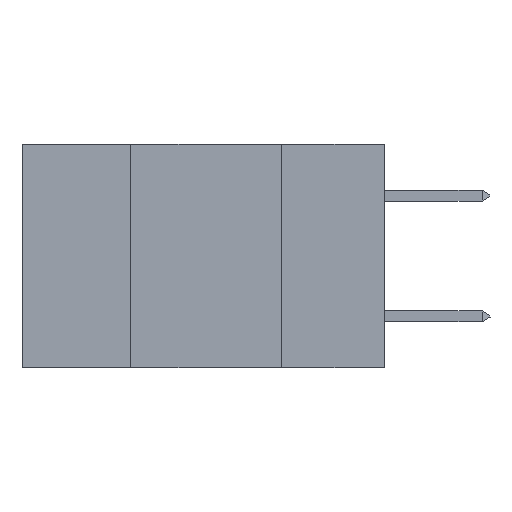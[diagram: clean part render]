
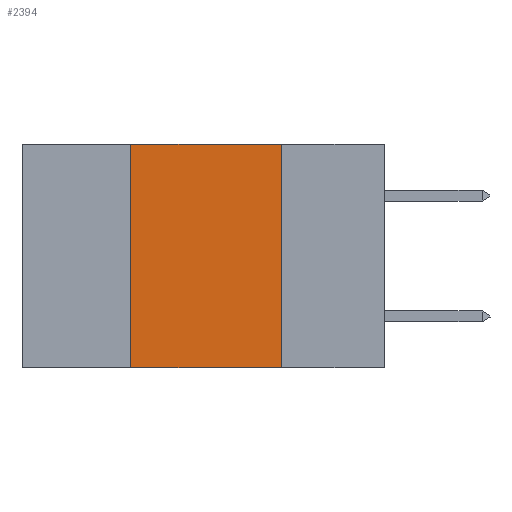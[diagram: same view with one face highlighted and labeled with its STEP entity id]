
A CAD part, left-side view. The second image highlights one B-rep face of the part: STEP entity #2394.
In plain terms, the highlighted planar face has unit normal (-1, 0, 0).
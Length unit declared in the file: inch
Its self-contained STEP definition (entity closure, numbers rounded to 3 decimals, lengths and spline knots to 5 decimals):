
#3 = DIRECTION ( 'NONE',  ( 0., 0., -1. ) ) ;
#60 = CARTESIAN_POINT ( 'NONE',  ( 0., 0.17, 0. ) ) ;
#2258 = VECTOR ( 'NONE', #3, 39.37008 ) ;
#2394 = ADVANCED_FACE ( 'NONE', ( #9257 ), #2480, .F. ) ;
#2465 = LINE ( 'NONE', #6908, #2258 ) ;
#2480 = PLANE ( 'NONE',  #5663 ) ;
#2553 = CARTESIAN_POINT ( 'NONE',  ( 0., 0.6, -0.37 ) ) ;
#2788 = CARTESIAN_POINT ( 'NONE',  ( 0., 0.6, 0. ) ) ;
#3071 = ORIENTED_EDGE ( 'NONE', *, *, #9585, .T. ) ;
#3486 = VECTOR ( 'NONE', #16187, 39.37008 ) ;
#3816 = DIRECTION ( 'NONE',  ( 1., 0., 0. ) ) ;
#3879 = EDGE_CURVE ( 'NONE', #3886, #11645, #2465, .T. ) ;
#3886 = VERTEX_POINT ( 'NONE', #60 ) ;
#4186 = VERTEX_POINT ( 'NONE', #7165 ) ;
#4314 = ORIENTED_EDGE ( 'NONE', *, *, #3879, .F. ) ;
#4969 = CARTESIAN_POINT ( 'NONE',  ( 0., 0.6, 0. ) ) ;
#5663 = AXIS2_PLACEMENT_3D ( 'NONE', #4969, #3816, #14661 ) ;
#6252 = LINE ( 'NONE', #9600, #3486 ) ;
#6908 = CARTESIAN_POINT ( 'NONE',  ( 0., 0.17, 0. ) ) ;
#7165 = CARTESIAN_POINT ( 'NONE',  ( 0., 0.42, 0. ) ) ;
#8088 = EDGE_CURVE ( 'NONE', #4186, #3886, #13004, .T. ) ;
#8935 = VECTOR ( 'NONE', #14752, 39.37008 ) ;
#9257 = FACE_OUTER_BOUND ( 'NONE', #10225, .T. ) ;
#9585 = EDGE_CURVE ( 'NONE', #10633, #11645, #17132, .T. ) ;
#9600 = CARTESIAN_POINT ( 'NONE',  ( 0., 0.42, 0. ) ) ;
#10225 = EDGE_LOOP ( 'NONE', ( #4314, #10701, #16729, #3071 ) ) ;
#10485 = VECTOR ( 'NONE', #14908, 39.37008 ) ;
#10633 = VERTEX_POINT ( 'NONE', #15061 ) ;
#10701 = ORIENTED_EDGE ( 'NONE', *, *, #8088, .F. ) ;
#11645 = VERTEX_POINT ( 'NONE', #17559 ) ;
#11876 = EDGE_CURVE ( 'NONE', #10633, #4186, #6252, .T. ) ;
#13004 = LINE ( 'NONE', #2788, #8935 ) ;
#14661 = DIRECTION ( 'NONE',  ( 0., 0., -1. ) ) ;
#14752 = DIRECTION ( 'NONE',  ( 0., -1., 0. ) ) ;
#14908 = DIRECTION ( 'NONE',  ( 0., -1., 0. ) ) ;
#15061 = CARTESIAN_POINT ( 'NONE',  ( 0., 0.42, -0.37 ) ) ;
#16187 = DIRECTION ( 'NONE',  ( 0., 0., 1. ) ) ;
#16729 = ORIENTED_EDGE ( 'NONE', *, *, #11876, .F. ) ;
#17132 = LINE ( 'NONE', #2553, #10485 ) ;
#17559 = CARTESIAN_POINT ( 'NONE',  ( 0., 0.17, -0.37 ) ) ;
